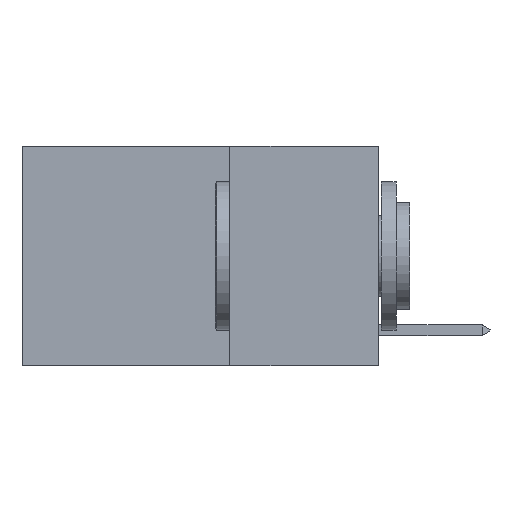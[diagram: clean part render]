
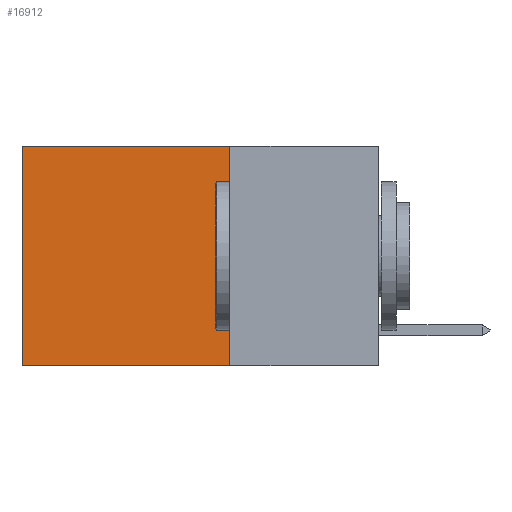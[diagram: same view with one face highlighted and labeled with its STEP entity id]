
A CAD part, left-side view. The second image highlights one B-rep face of the part: STEP entity #16912.
In plain terms, the highlighted planar face has unit normal (-1, 0, 0).
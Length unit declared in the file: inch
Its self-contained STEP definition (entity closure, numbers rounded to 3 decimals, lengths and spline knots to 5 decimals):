
#440 = CARTESIAN_POINT ( 'NONE',  ( 0.2625, 0.6, -0.37 ) ) ;
#507 = CARTESIAN_POINT ( 'NONE',  ( 0.2625, 0.25, 0. ) ) ;
#1037 = EDGE_LOOP ( 'NONE', ( #4307, #8640, #6144, #14846 ) ) ;
#1368 = VERTEX_POINT ( 'NONE', #10421 ) ;
#1532 = EDGE_CURVE ( 'NONE', #6317, #1368, #18329, .T. ) ;
#1571 = LINE ( 'NONE', #16080, #7837 ) ;
#1955 = DIRECTION ( 'NONE',  ( 0., 0., -1. ) ) ;
#3386 = PLANE ( 'NONE',  #13797 ) ;
#4307 = ORIENTED_EDGE ( 'NONE', *, *, #15811, .T. ) ;
#5931 = VERTEX_POINT ( 'NONE', #440 ) ;
#6144 = ORIENTED_EDGE ( 'NONE', *, *, #12725, .F. ) ;
#6317 = VERTEX_POINT ( 'NONE', #13956 ) ;
#6405 = VECTOR ( 'NONE', #16138, 39.37008 ) ;
#7484 = LINE ( 'NONE', #11785, #6405 ) ;
#7837 = VECTOR ( 'NONE', #17429, 39.37008 ) ;
#8640 = ORIENTED_EDGE ( 'NONE', *, *, #9051, .F. ) ;
#8987 = LINE ( 'NONE', #9078, #9721 ) ;
#9051 = EDGE_CURVE ( 'NONE', #10952, #5931, #1571, .T. ) ;
#9078 = CARTESIAN_POINT ( 'NONE',  ( 0.2625, 0.25, 0. ) ) ;
#9565 = DIRECTION ( 'NONE',  ( 0., 1., 0. ) ) ;
#9721 = VECTOR ( 'NONE', #13697, 39.37008 ) ;
#10026 = VECTOR ( 'NONE', #9565, 39.37008 ) ;
#10054 = CARTESIAN_POINT ( 'NONE',  ( 0.2625, 0.25, -0.37 ) ) ;
#10421 = CARTESIAN_POINT ( 'NONE',  ( 0.2625, 0.6, 0. ) ) ;
#10655 = FACE_OUTER_BOUND ( 'NONE', #1037, .T. ) ;
#10952 = VERTEX_POINT ( 'NONE', #10054 ) ;
#11785 = CARTESIAN_POINT ( 'NONE',  ( 0.2625, 0.6, 0. ) ) ;
#12725 = EDGE_CURVE ( 'NONE', #6317, #10952, #8987, .T. ) ;
#13697 = DIRECTION ( 'NONE',  ( 0., 0., -1. ) ) ;
#13797 = AXIS2_PLACEMENT_3D ( 'NONE', #507, #15103, #1955 ) ;
#13956 = CARTESIAN_POINT ( 'NONE',  ( 0.2625, 0.25, 0. ) ) ;
#14077 = CARTESIAN_POINT ( 'NONE',  ( 0.2625, 0.25, 0. ) ) ;
#14846 = ORIENTED_EDGE ( 'NONE', *, *, #1532, .T. ) ;
#15103 = DIRECTION ( 'NONE',  ( 1., 0., 0. ) ) ;
#15811 = EDGE_CURVE ( 'NONE', #1368, #5931, #7484, .T. ) ;
#16080 = CARTESIAN_POINT ( 'NONE',  ( 0.2625, 0.25, -0.37 ) ) ;
#16138 = DIRECTION ( 'NONE',  ( 0., 0., -1. ) ) ;
#16912 = ADVANCED_FACE ( 'NONE', ( #10655 ), #3386, .F. ) ;
#17429 = DIRECTION ( 'NONE',  ( 0., 1., 0. ) ) ;
#18329 = LINE ( 'NONE', #14077, #10026 ) ;
